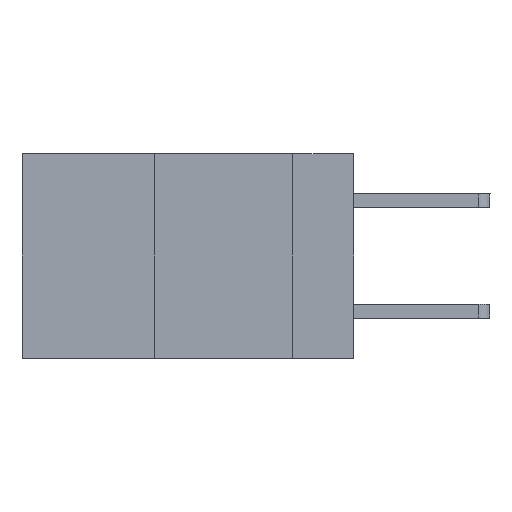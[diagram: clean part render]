
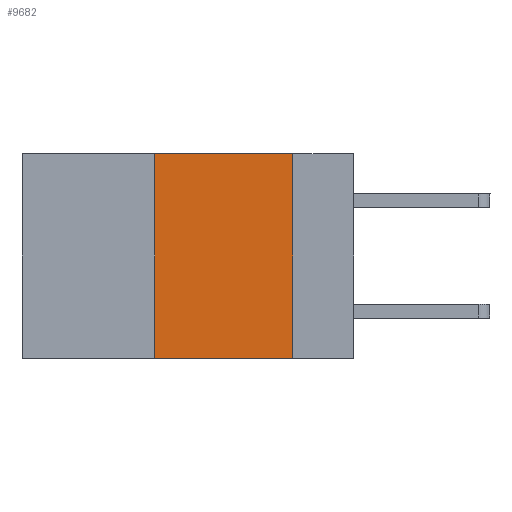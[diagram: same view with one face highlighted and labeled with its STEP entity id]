
A CAD part, left-side view. The second image highlights one B-rep face of the part: STEP entity #9682.
In plain terms, the highlighted planar face has unit normal (-1, 0, 0).
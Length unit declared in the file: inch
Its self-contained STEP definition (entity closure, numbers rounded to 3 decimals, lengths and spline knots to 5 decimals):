
#26 = CARTESIAN_POINT ( 'NONE',  ( 0., 0.36, -0.37 ) ) ;
#469 = VERTEX_POINT ( 'NONE', #26 ) ;
#1239 = ORIENTED_EDGE ( 'NONE', *, *, #5190, .F. ) ;
#1408 = VECTOR ( 'NONE', #4139, 39.37008 ) ;
#1497 = VECTOR ( 'NONE', #9414, 39.37008 ) ;
#1814 = PLANE ( 'NONE',  #13818 ) ;
#1865 = VERTEX_POINT ( 'NONE', #6291 ) ;
#1990 = ORIENTED_EDGE ( 'NONE', *, *, #7643, .F. ) ;
#2829 = DIRECTION ( 'NONE',  ( 0., -1., 0. ) ) ;
#4139 = DIRECTION ( 'NONE',  ( 0., -1., 0. ) ) ;
#4155 = CARTESIAN_POINT ( 'NONE',  ( 0., 0.6, -0.37 ) ) ;
#4635 = LINE ( 'NONE', #12490, #1497 ) ;
#5190 = EDGE_CURVE ( 'NONE', #7315, #1865, #8150, .T. ) ;
#5304 = CARTESIAN_POINT ( 'NONE',  ( 0., 0.6, 0. ) ) ;
#5351 = DIRECTION ( 'NONE',  ( 1., 0., 0. ) ) ;
#6151 = EDGE_CURVE ( 'NONE', #469, #1865, #10259, .T. ) ;
#6291 = CARTESIAN_POINT ( 'NONE',  ( 0., 0.11, -0.37 ) ) ;
#7315 = VERTEX_POINT ( 'NONE', #11990 ) ;
#7583 = VECTOR ( 'NONE', #2829, 39.37008 ) ;
#7643 = EDGE_CURVE ( 'NONE', #9631, #7315, #7926, .T. ) ;
#7926 = LINE ( 'NONE', #9371, #7583 ) ;
#7978 = DIRECTION ( 'NONE',  ( 0., 0., -1. ) ) ;
#8065 = CARTESIAN_POINT ( 'NONE',  ( 0., 0.11, 0. ) ) ;
#8150 = LINE ( 'NONE', #8065, #13326 ) ;
#8339 = EDGE_LOOP ( 'NONE', ( #1239, #1990, #8527, #9008 ) ) ;
#8527 = ORIENTED_EDGE ( 'NONE', *, *, #10828, .F. ) ;
#9008 = ORIENTED_EDGE ( 'NONE', *, *, #6151, .T. ) ;
#9371 = CARTESIAN_POINT ( 'NONE',  ( 0., 0.6, 0. ) ) ;
#9414 = DIRECTION ( 'NONE',  ( 0., 0., 1. ) ) ;
#9631 = VERTEX_POINT ( 'NONE', #13574 ) ;
#9682 = ADVANCED_FACE ( 'NONE', ( #13356 ), #1814, .F. ) ;
#10259 = LINE ( 'NONE', #4155, #1408 ) ;
#10828 = EDGE_CURVE ( 'NONE', #469, #9631, #4635, .T. ) ;
#11990 = CARTESIAN_POINT ( 'NONE',  ( 0., 0.11, 0. ) ) ;
#12490 = CARTESIAN_POINT ( 'NONE',  ( 0., 0.36, 0. ) ) ;
#12692 = DIRECTION ( 'NONE',  ( 0., 0., -1. ) ) ;
#13326 = VECTOR ( 'NONE', #7978, 39.37008 ) ;
#13356 = FACE_OUTER_BOUND ( 'NONE', #8339, .T. ) ;
#13574 = CARTESIAN_POINT ( 'NONE',  ( 0., 0.36, 0. ) ) ;
#13818 = AXIS2_PLACEMENT_3D ( 'NONE', #5304, #5351, #12692 ) ;
